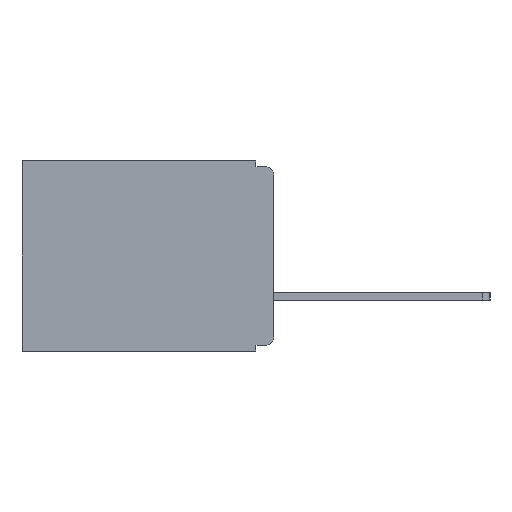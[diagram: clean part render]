
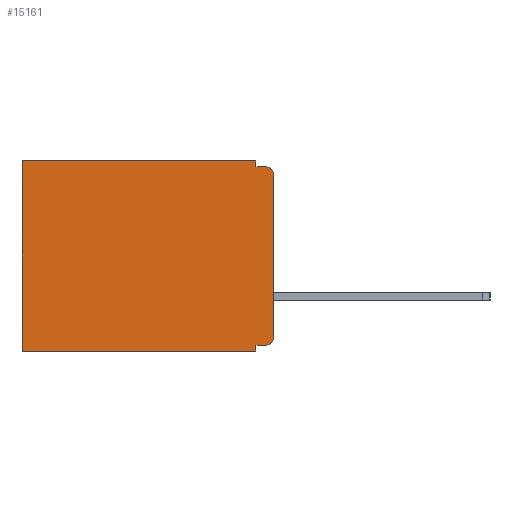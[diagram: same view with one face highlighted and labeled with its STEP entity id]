
A CAD part, left-side view. The second image highlights one B-rep face of the part: STEP entity #15161.
In plain terms, the highlighted planar face has unit normal (-1, 0, 0).
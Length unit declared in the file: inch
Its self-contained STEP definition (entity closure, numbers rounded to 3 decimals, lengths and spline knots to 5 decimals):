
#83 = DIRECTION ( 'NONE',  ( 0., 1., 0. ) ) ;
#139 = VERTEX_POINT ( 'NONE', #5720 ) ;
#203 = DIRECTION ( 'NONE',  ( 0., 0., -1. ) ) ;
#226 = CARTESIAN_POINT ( 'NONE',  ( 0.3, 0.015, -0.01 ) ) ;
#234 = DIRECTION ( 'NONE',  ( 0., 0., -1. ) ) ;
#430 = VERTEX_POINT ( 'NONE', #4201 ) ;
#599 = ORIENTED_EDGE ( 'NONE', *, *, #22117, .F. ) ;
#1213 = ORIENTED_EDGE ( 'NONE', *, *, #19788, .F. ) ;
#1268 = VECTOR ( 'NONE', #9365, 39.37008 ) ;
#1317 = VERTEX_POINT ( 'NONE', #19054 ) ;
#1566 = VERTEX_POINT ( 'NONE', #20048 ) ;
#1968 = EDGE_LOOP ( 'NONE', ( #599, #9420, #17074, #14414, #21441, #14545, #1213, #5187, #15317, #2026 ) ) ;
#2026 = ORIENTED_EDGE ( 'NONE', *, *, #14781, .T. ) ;
#2061 = CARTESIAN_POINT ( 'NONE',  ( 0.3, 0., -0.32 ) ) ;
#2199 = EDGE_CURVE ( 'NONE', #12099, #19087, #12829, .T. ) ;
#3367 = DIRECTION ( 'NONE',  ( 1., 0., 0. ) ) ;
#3404 = VECTOR ( 'NONE', #203, 39.37008 ) ;
#4201 = CARTESIAN_POINT ( 'NONE',  ( 0.3, 0.437, -0.33 ) ) ;
#4519 = VERTEX_POINT ( 'NONE', #19561 ) ;
#4587 = CARTESIAN_POINT ( 'NONE',  ( 0.3, 0., -0.305 ) ) ;
#4732 = LINE ( 'NONE', #2061, #17822 ) ;
#4906 = CARTESIAN_POINT ( 'NONE',  ( 0.3, 0.031, -0.01 ) ) ;
#5052 = EDGE_CURVE ( 'NONE', #1566, #12099, #8611, .T. ) ;
#5187 = ORIENTED_EDGE ( 'NONE', *, *, #12053, .F. ) ;
#5370 = VECTOR ( 'NONE', #23922, 39.37008 ) ;
#5378 = CARTESIAN_POINT ( 'NONE',  ( 0.3, 0., -0.33 ) ) ;
#5411 = VECTOR ( 'NONE', #16424, 39.37008 ) ;
#5720 = CARTESIAN_POINT ( 'NONE',  ( 0.3, 0.031, -0.33 ) ) ;
#6270 = CARTESIAN_POINT ( 'NONE',  ( 0.3, 0., -0.025 ) ) ;
#7312 = DIRECTION ( 'NONE',  ( 0., 0., -1. ) ) ;
#7997 = FACE_OUTER_BOUND ( 'NONE', #1968, .T. ) ;
#8100 = CARTESIAN_POINT ( 'NONE',  ( 0.3, 0.015, -0.305 ) ) ;
#8609 = CIRCLE ( 'NONE', #19183, 0.015 ) ;
#8611 = LINE ( 'NONE', #15606, #3404 ) ;
#8681 = CARTESIAN_POINT ( 'NONE',  ( 0.3, 0.031, -0.33 ) ) ;
#8740 = CARTESIAN_POINT ( 'NONE',  ( 0.3, 0., 0. ) ) ;
#9365 = DIRECTION ( 'NONE',  ( 0., -1., 0. ) ) ;
#9420 = ORIENTED_EDGE ( 'NONE', *, *, #24023, .T. ) ;
#10047 = DIRECTION ( 'NONE',  ( 0., 0., -1. ) ) ;
#10266 = LINE ( 'NONE', #8740, #14805 ) ;
#11045 = CARTESIAN_POINT ( 'NONE',  ( 0.3, 0., -0.33 ) ) ;
#11132 = AXIS2_PLACEMENT_3D ( 'NONE', #11045, #3367, #17034 ) ;
#11161 = LINE ( 'NONE', #22029, #5370 ) ;
#11903 = DIRECTION ( 'NONE',  ( -1., 0., 0. ) ) ;
#12053 = EDGE_CURVE ( 'NONE', #4519, #139, #15758, .T. ) ;
#12099 = VERTEX_POINT ( 'NONE', #4906 ) ;
#12561 = CARTESIAN_POINT ( 'NONE',  ( 0.3, 0., -0.01 ) ) ;
#12715 = EDGE_CURVE ( 'NONE', #1566, #1317, #10266, .T. ) ;
#12829 = LINE ( 'NONE', #12561, #1268 ) ;
#12910 = VERTEX_POINT ( 'NONE', #22925 ) ;
#13107 = VERTEX_POINT ( 'NONE', #4587 ) ;
#13205 = LINE ( 'NONE', #5378, #17212 ) ;
#14414 = ORIENTED_EDGE ( 'NONE', *, *, #5052, .F. ) ;
#14545 = ORIENTED_EDGE ( 'NONE', *, *, #23222, .T. ) ;
#14576 = DIRECTION ( 'NONE',  ( 0., 1., 0. ) ) ;
#14781 = EDGE_CURVE ( 'NONE', #12910, #13107, #17157, .T. ) ;
#14805 = VECTOR ( 'NONE', #14576, 39.37008 ) ;
#15161 = ADVANCED_FACE ( 'NONE', ( #7997 ), #22802, .F. ) ;
#15317 = ORIENTED_EDGE ( 'NONE', *, *, #20310, .F. ) ;
#15485 = VERTEX_POINT ( 'NONE', #6270 ) ;
#15606 = CARTESIAN_POINT ( 'NONE',  ( 0.3, 0.031, 0. ) ) ;
#15758 = LINE ( 'NONE', #8681, #5411 ) ;
#15959 = VECTOR ( 'NONE', #7312, 39.37008 ) ;
#16424 = DIRECTION ( 'NONE',  ( 0., 0., -1. ) ) ;
#17034 = DIRECTION ( 'NONE',  ( 0., 0., -1. ) ) ;
#17074 = ORIENTED_EDGE ( 'NONE', *, *, #2199, .F. ) ;
#17157 = CIRCLE ( 'NONE', #22554, 0.015 ) ;
#17212 = VECTOR ( 'NONE', #24726, 39.37008 ) ;
#17822 = VECTOR ( 'NONE', #83, 39.37008 ) ;
#19054 = CARTESIAN_POINT ( 'NONE',  ( 0.3, 0.437, 0. ) ) ;
#19087 = VERTEX_POINT ( 'NONE', #226 ) ;
#19183 = AXIS2_PLACEMENT_3D ( 'NONE', #23543, #11903, #234 ) ;
#19561 = CARTESIAN_POINT ( 'NONE',  ( 0.3, 0.031, -0.32 ) ) ;
#19788 = EDGE_CURVE ( 'NONE', #139, #430, #11161, .T. ) ;
#20048 = CARTESIAN_POINT ( 'NONE',  ( 0.3, 0.031, 0. ) ) ;
#20310 = EDGE_CURVE ( 'NONE', #12910, #4519, #4732, .T. ) ;
#20934 = CARTESIAN_POINT ( 'NONE',  ( 0.3, 0.437, -0.33 ) ) ;
#21441 = ORIENTED_EDGE ( 'NONE', *, *, #12715, .T. ) ;
#21724 = DIRECTION ( 'NONE',  ( -1., 0., 0. ) ) ;
#21757 = LINE ( 'NONE', #20934, #15959 ) ;
#22029 = CARTESIAN_POINT ( 'NONE',  ( 0.3, 0., -0.33 ) ) ;
#22117 = EDGE_CURVE ( 'NONE', #15485, #13107, #13205, .T. ) ;
#22554 = AXIS2_PLACEMENT_3D ( 'NONE', #8100, #21724, #10047 ) ;
#22802 = PLANE ( 'NONE',  #11132 ) ;
#22925 = CARTESIAN_POINT ( 'NONE',  ( 0.3, 0.015, -0.32 ) ) ;
#23222 = EDGE_CURVE ( 'NONE', #1317, #430, #21757, .T. ) ;
#23543 = CARTESIAN_POINT ( 'NONE',  ( 0.3, 0.015, -0.025 ) ) ;
#23922 = DIRECTION ( 'NONE',  ( 0., 1., 0. ) ) ;
#24023 = EDGE_CURVE ( 'NONE', #15485, #19087, #8609, .T. ) ;
#24726 = DIRECTION ( 'NONE',  ( 0., 0., -1. ) ) ;
